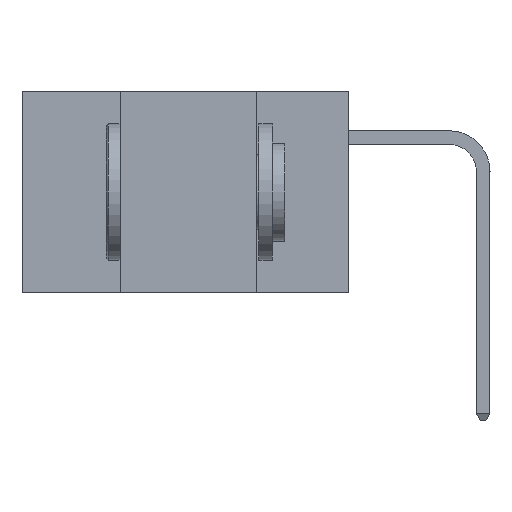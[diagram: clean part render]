
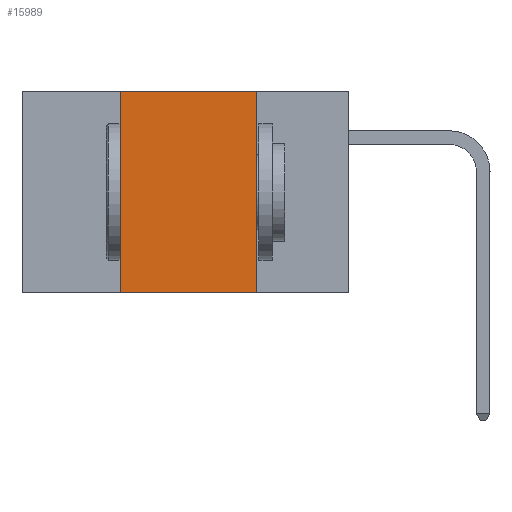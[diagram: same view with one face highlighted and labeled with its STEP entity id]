
A CAD part, left-side view. The second image highlights one B-rep face of the part: STEP entity #15989.
In plain terms, the highlighted planar face has unit normal (-1, 0, 0).
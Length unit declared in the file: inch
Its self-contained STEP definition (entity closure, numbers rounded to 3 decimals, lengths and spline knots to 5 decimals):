
#2379 = DIRECTION ( 'NONE',  ( 0., 0., -1. ) ) ;
#5504 = VECTOR ( 'NONE', #41119, 39.37008 ) ;
#6140 = VECTOR ( 'NONE', #13580, 39.37008 ) ;
#7156 = VERTEX_POINT ( 'NONE', #37269 ) ;
#8128 = DIRECTION ( 'NONE',  ( 1., 0., 0. ) ) ;
#12745 = CARTESIAN_POINT ( 'NONE',  ( 0., 0.42, 0. ) ) ;
#13580 = DIRECTION ( 'NONE',  ( 0., -1., 0. ) ) ;
#14276 = VECTOR ( 'NONE', #2379, 39.37008 ) ;
#14340 = VERTEX_POINT ( 'NONE', #42764 ) ;
#15989 = ADVANCED_FACE ( 'NONE', ( #43594 ), #28354, .F. ) ;
#16420 = CARTESIAN_POINT ( 'NONE',  ( 0., 0.17, 0. ) ) ;
#16472 = EDGE_LOOP ( 'NONE', ( #39357, #27295, #42119, #18480 ) ) ;
#18480 = ORIENTED_EDGE ( 'NONE', *, *, #45724, .T. ) ;
#19408 = VERTEX_POINT ( 'NONE', #32243 ) ;
#20967 = LINE ( 'NONE', #16420, #14276 ) ;
#21101 = LINE ( 'NONE', #12745, #5504 ) ;
#21364 = DIRECTION ( 'NONE',  ( 0., 0., -1. ) ) ;
#24736 = CARTESIAN_POINT ( 'NONE',  ( 0., 0.6, 0. ) ) ;
#26306 = CARTESIAN_POINT ( 'NONE',  ( 0., 0.42, 0. ) ) ;
#27295 = ORIENTED_EDGE ( 'NONE', *, *, #30048, .F. ) ;
#28354 = PLANE ( 'NONE',  #29650 ) ;
#29650 = AXIS2_PLACEMENT_3D ( 'NONE', #40096, #8128, #21364 ) ;
#30048 = EDGE_CURVE ( 'NONE', #34913, #19408, #31161, .T. ) ;
#30538 = EDGE_CURVE ( 'NONE', #14340, #34913, #21101, .T. ) ;
#31161 = LINE ( 'NONE', #24736, #6140 ) ;
#32243 = CARTESIAN_POINT ( 'NONE',  ( 0., 0.17, 0. ) ) ;
#32245 = EDGE_CURVE ( 'NONE', #19408, #7156, #20967, .T. ) ;
#33178 = VECTOR ( 'NONE', #40289, 39.37008 ) ;
#34913 = VERTEX_POINT ( 'NONE', #26306 ) ;
#37189 = CARTESIAN_POINT ( 'NONE',  ( 0., 0.6, -0.37 ) ) ;
#37269 = CARTESIAN_POINT ( 'NONE',  ( 0., 0.17, -0.37 ) ) ;
#39357 = ORIENTED_EDGE ( 'NONE', *, *, #32245, .F. ) ;
#40096 = CARTESIAN_POINT ( 'NONE',  ( 0., 0.6, 0. ) ) ;
#40289 = DIRECTION ( 'NONE',  ( 0., -1., 0. ) ) ;
#41119 = DIRECTION ( 'NONE',  ( 0., 0., 1. ) ) ;
#42119 = ORIENTED_EDGE ( 'NONE', *, *, #30538, .F. ) ;
#42627 = LINE ( 'NONE', #37189, #33178 ) ;
#42764 = CARTESIAN_POINT ( 'NONE',  ( 0., 0.42, -0.37 ) ) ;
#43594 = FACE_OUTER_BOUND ( 'NONE', #16472, .T. ) ;
#45724 = EDGE_CURVE ( 'NONE', #14340, #7156, #42627, .T. ) ;
